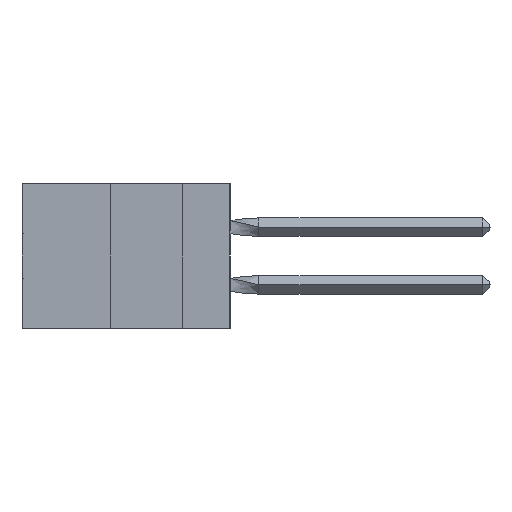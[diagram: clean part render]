
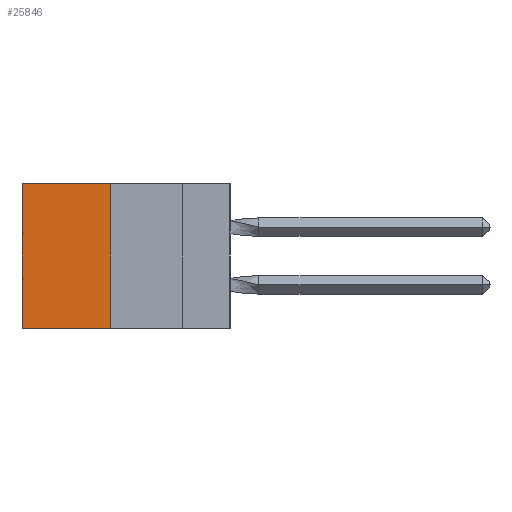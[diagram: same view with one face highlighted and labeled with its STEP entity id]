
A CAD part, left-side view. The second image highlights one B-rep face of the part: STEP entity #25846.
In plain terms, the highlighted planar face has unit normal (-1, 0, 0).
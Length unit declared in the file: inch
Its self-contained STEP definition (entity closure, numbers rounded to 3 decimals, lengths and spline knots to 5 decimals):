
#222 = VERTEX_POINT ( 'NONE', #38252 ) ;
#1295 = DIRECTION ( 'NONE',  ( 0., 0., -1. ) ) ;
#2014 = ORIENTED_EDGE ( 'NONE', *, *, #44483, .F. ) ;
#2717 = ORIENTED_EDGE ( 'NONE', *, *, #22684, .F. ) ;
#4047 = VERTEX_POINT ( 'NONE', #46013 ) ;
#4512 = CARTESIAN_POINT ( 'NONE',  ( 0.305, 0.413, -0.5 ) ) ;
#4546 = VERTEX_POINT ( 'NONE', #26280 ) ;
#5985 = DIRECTION ( 'NONE',  ( 0., 0., -1. ) ) ;
#8119 = DIRECTION ( 'NONE',  ( 0., 0., -1. ) ) ;
#8963 = DIRECTION ( 'NONE',  ( 0., 1., 0. ) ) ;
#12662 = VECTOR ( 'NONE', #8119, 39.37008 ) ;
#12698 = CARTESIAN_POINT ( 'NONE',  ( 0.305, 0.413, -0.5 ) ) ;
#13185 = DIRECTION ( 'NONE',  ( 1., 0., 0. ) ) ;
#15577 = DIRECTION ( 'NONE',  ( 0., 1., 0. ) ) ;
#19841 = VECTOR ( 'NONE', #8963, 39.37008 ) ;
#21389 = EDGE_LOOP ( 'NONE', ( #38078, #2014, #2717, #37475 ) ) ;
#22684 = EDGE_CURVE ( 'NONE', #4546, #27138, #27854, .T. ) ;
#25846 = ADVANCED_FACE ( 'NONE', ( #34675 ), #31844, .F. ) ;
#26280 = CARTESIAN_POINT ( 'NONE',  ( 0.305, 0.413, 0. ) ) ;
#27138 = VERTEX_POINT ( 'NONE', #4512 ) ;
#27854 = LINE ( 'NONE', #43798, #46761 ) ;
#31162 = CARTESIAN_POINT ( 'NONE',  ( 0.305, 0.72, -0.5 ) ) ;
#31844 = PLANE ( 'NONE',  #46711 ) ;
#32771 = LINE ( 'NONE', #31162, #12662 ) ;
#34675 = FACE_OUTER_BOUND ( 'NONE', #21389, .T. ) ;
#37217 = VECTOR ( 'NONE', #15577, 39.37008 ) ;
#37475 = ORIENTED_EDGE ( 'NONE', *, *, #48364, .T. ) ;
#38078 = ORIENTED_EDGE ( 'NONE', *, *, #43122, .T. ) ;
#38244 = CARTESIAN_POINT ( 'NONE',  ( 0.305, 0.413, 0. ) ) ;
#38252 = CARTESIAN_POINT ( 'NONE',  ( 0.305, 0.72, -0.5 ) ) ;
#38395 = LINE ( 'NONE', #38244, #37217 ) ;
#39921 = LINE ( 'NONE', #43142, #19841 ) ;
#43122 = EDGE_CURVE ( 'NONE', #4047, #222, #32771, .T. ) ;
#43142 = CARTESIAN_POINT ( 'NONE',  ( 0.305, 0.413, -0.5 ) ) ;
#43798 = CARTESIAN_POINT ( 'NONE',  ( 0.305, 0.413, -0.5 ) ) ;
#44483 = EDGE_CURVE ( 'NONE', #27138, #222, #39921, .T. ) ;
#46013 = CARTESIAN_POINT ( 'NONE',  ( 0.305, 0.72, 0. ) ) ;
#46711 = AXIS2_PLACEMENT_3D ( 'NONE', #12698, #13185, #1295 ) ;
#46761 = VECTOR ( 'NONE', #5985, 39.37008 ) ;
#48364 = EDGE_CURVE ( 'NONE', #4546, #4047, #38395, .T. ) ;
